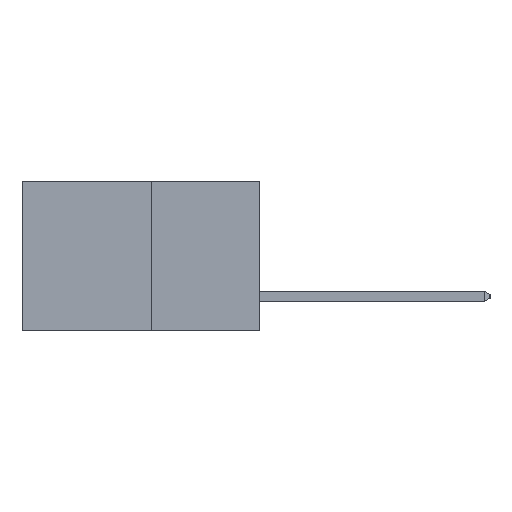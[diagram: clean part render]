
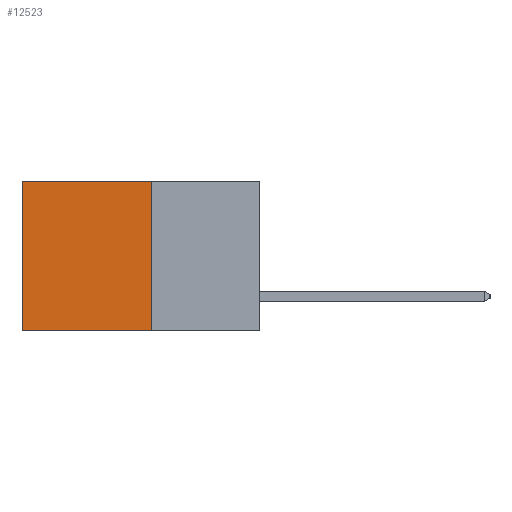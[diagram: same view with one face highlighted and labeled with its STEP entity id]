
A CAD part, left-side view. The second image highlights one B-rep face of the part: STEP entity #12523.
In plain terms, the highlighted planar face has unit normal (-1, 0, 0).
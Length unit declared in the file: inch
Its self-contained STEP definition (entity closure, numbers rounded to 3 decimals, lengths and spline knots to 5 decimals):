
#899 = VERTEX_POINT ( 'NONE', #1537 ) ;
#1345 = ORIENTED_EDGE ( 'NONE', *, *, #8899, .T. ) ;
#1502 = CARTESIAN_POINT ( 'NONE',  ( 0.277, 0.27, 0. ) ) ;
#1537 = CARTESIAN_POINT ( 'NONE',  ( 0.277, 0.27, -0.37 ) ) ;
#2792 = CARTESIAN_POINT ( 'NONE',  ( 0.277, 0.59, -0.37 ) ) ;
#2901 = CARTESIAN_POINT ( 'NONE',  ( 0.277, 0.59, -0.37 ) ) ;
#3314 = ORIENTED_EDGE ( 'NONE', *, *, #13630, .T. ) ;
#4669 = LINE ( 'NONE', #17229, #28096 ) ;
#5910 = ORIENTED_EDGE ( 'NONE', *, *, #21291, .F. ) ;
#7733 = CARTESIAN_POINT ( 'NONE',  ( 0.277, 0.27, -0.37 ) ) ;
#8899 = EDGE_CURVE ( 'NONE', #21136, #13683, #4669, .T. ) ;
#9383 = FACE_OUTER_BOUND ( 'NONE', #24169, .T. ) ;
#10011 = DIRECTION ( 'NONE',  ( 0., 0., -1. ) ) ;
#12523 = ADVANCED_FACE ( 'NONE', ( #9383 ), #16808, .F. ) ;
#12717 = DIRECTION ( 'NONE',  ( 0., 1., 0. ) ) ;
#13630 = EDGE_CURVE ( 'NONE', #13683, #19652, #25369, .T. ) ;
#13683 = VERTEX_POINT ( 'NONE', #27906 ) ;
#13720 = CARTESIAN_POINT ( 'NONE',  ( 0.277, 0.27, -0.37 ) ) ;
#14725 = VECTOR ( 'NONE', #18764, 39.37008 ) ;
#16808 = PLANE ( 'NONE',  #25514 ) ;
#16925 = EDGE_CURVE ( 'NONE', #21136, #899, #18095, .T. ) ;
#17229 = CARTESIAN_POINT ( 'NONE',  ( 0.277, 0.27, 0. ) ) ;
#17982 = DIRECTION ( 'NONE',  ( 0., 1., 0. ) ) ;
#18095 = LINE ( 'NONE', #13720, #29306 ) ;
#18764 = DIRECTION ( 'NONE',  ( 0., 0., -1. ) ) ;
#19652 = VERTEX_POINT ( 'NONE', #2901 ) ;
#20019 = LINE ( 'NONE', #29143, #26721 ) ;
#20618 = DIRECTION ( 'NONE',  ( 0., 0., -1. ) ) ;
#21136 = VERTEX_POINT ( 'NONE', #1502 ) ;
#21291 = EDGE_CURVE ( 'NONE', #899, #19652, #20019, .T. ) ;
#21881 = ORIENTED_EDGE ( 'NONE', *, *, #16925, .F. ) ;
#23652 = DIRECTION ( 'NONE',  ( 1., 0., 0. ) ) ;
#24169 = EDGE_LOOP ( 'NONE', ( #3314, #5910, #21881, #1345 ) ) ;
#25369 = LINE ( 'NONE', #2792, #14725 ) ;
#25514 = AXIS2_PLACEMENT_3D ( 'NONE', #7733, #23652, #10011 ) ;
#26721 = VECTOR ( 'NONE', #17982, 39.37008 ) ;
#27906 = CARTESIAN_POINT ( 'NONE',  ( 0.277, 0.59, 0. ) ) ;
#28096 = VECTOR ( 'NONE', #12717, 39.37008 ) ;
#29143 = CARTESIAN_POINT ( 'NONE',  ( 0.277, 0.27, -0.37 ) ) ;
#29306 = VECTOR ( 'NONE', #20618, 39.37008 ) ;
